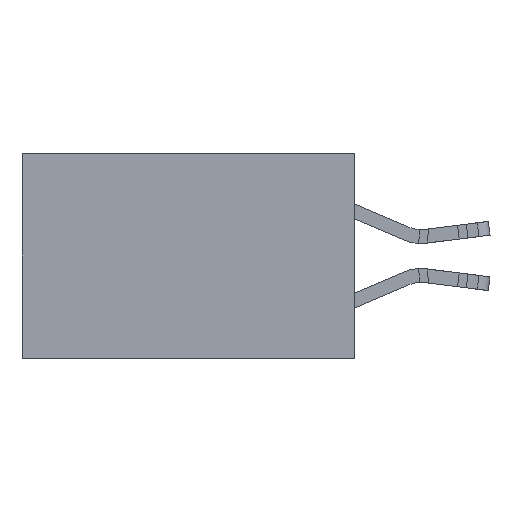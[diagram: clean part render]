
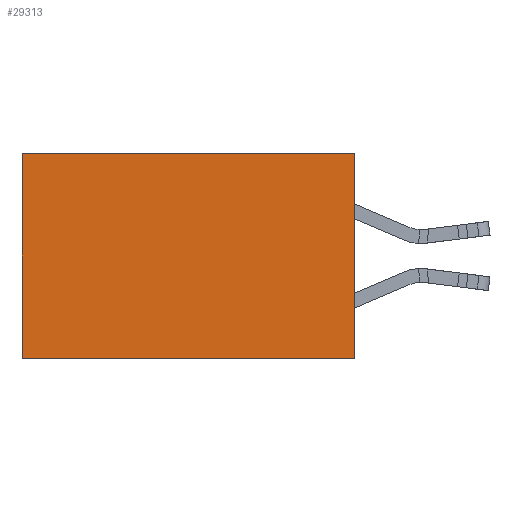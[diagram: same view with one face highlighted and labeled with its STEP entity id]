
A CAD part, left-side view. The second image highlights one B-rep face of the part: STEP entity #29313.
In plain terms, the highlighted planar face has unit normal (-1, 0, 0).
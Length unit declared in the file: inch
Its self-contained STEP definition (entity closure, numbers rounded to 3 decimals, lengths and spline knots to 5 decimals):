
#94 = CARTESIAN_POINT ( 'NONE',  ( 0.298, 0., 0. ) ) ;
#324 = ORIENTED_EDGE ( 'NONE', *, *, #24776, .F. ) ;
#897 = VECTOR ( 'NONE', #3126, 39.37008 ) ;
#2751 = EDGE_CURVE ( 'NONE', #8591, #22192, #13032, .T. ) ;
#3126 = DIRECTION ( 'NONE',  ( 0., 0., -1. ) ) ;
#3187 = FACE_OUTER_BOUND ( 'NONE', #19238, .T. ) ;
#3487 = VERTEX_POINT ( 'NONE', #29838 ) ;
#4764 = AXIS2_PLACEMENT_3D ( 'NONE', #94, #10227, #17708 ) ;
#4809 = DIRECTION ( 'NONE',  ( 0., 1., 0. ) ) ;
#7254 = ORIENTED_EDGE ( 'NONE', *, *, #2751, .T. ) ;
#8591 = VERTEX_POINT ( 'NONE', #11663 ) ;
#9035 = DIRECTION ( 'NONE',  ( 0., 0., -1. ) ) ;
#9172 = VECTOR ( 'NONE', #12008, 39.37008 ) ;
#10227 = DIRECTION ( 'NONE',  ( 1., 0., 0. ) ) ;
#11663 = CARTESIAN_POINT ( 'NONE',  ( 0.298, 0.6, 0. ) ) ;
#12008 = DIRECTION ( 'NONE',  ( 0., 1., 0. ) ) ;
#12035 = CARTESIAN_POINT ( 'NONE',  ( 0.298, 0., -0.37 ) ) ;
#12379 = CARTESIAN_POINT ( 'NONE',  ( 0.298, 0., -0.37 ) ) ;
#12645 = PLANE ( 'NONE',  #4764 ) ;
#13032 = LINE ( 'NONE', #14095, #24051 ) ;
#14095 = CARTESIAN_POINT ( 'NONE',  ( 0.298, 0.6, 0. ) ) ;
#14982 = ORIENTED_EDGE ( 'NONE', *, *, #16149, .F. ) ;
#15927 = VECTOR ( 'NONE', #4809, 39.37008 ) ;
#16149 = EDGE_CURVE ( 'NONE', #23106, #22192, #29320, .T. ) ;
#17446 = EDGE_CURVE ( 'NONE', #3487, #8591, #30014, .T. ) ;
#17708 = DIRECTION ( 'NONE',  ( 0., 0., -1. ) ) ;
#18634 = LINE ( 'NONE', #26187, #897 ) ;
#19238 = EDGE_LOOP ( 'NONE', ( #7254, #14982, #324, #22269 ) ) ;
#22192 = VERTEX_POINT ( 'NONE', #26372 ) ;
#22269 = ORIENTED_EDGE ( 'NONE', *, *, #17446, .T. ) ;
#23106 = VERTEX_POINT ( 'NONE', #12035 ) ;
#24051 = VECTOR ( 'NONE', #9035, 39.37008 ) ;
#24776 = EDGE_CURVE ( 'NONE', #3487, #23106, #18634, .T. ) ;
#26187 = CARTESIAN_POINT ( 'NONE',  ( 0.298, 0., 0. ) ) ;
#26372 = CARTESIAN_POINT ( 'NONE',  ( 0.298, 0.6, -0.37 ) ) ;
#29313 = ADVANCED_FACE ( 'NONE', ( #3187 ), #12645, .F. ) ;
#29320 = LINE ( 'NONE', #12379, #15927 ) ;
#29838 = CARTESIAN_POINT ( 'NONE',  ( 0.298, 0., 0. ) ) ;
#30014 = LINE ( 'NONE', #32160, #9172 ) ;
#32160 = CARTESIAN_POINT ( 'NONE',  ( 0.298, 0., 0. ) ) ;
